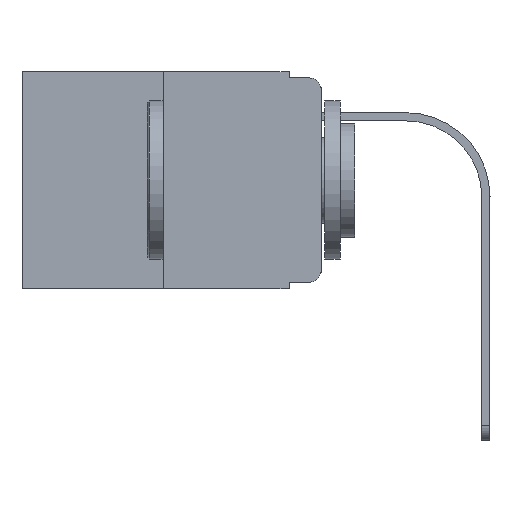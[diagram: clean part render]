
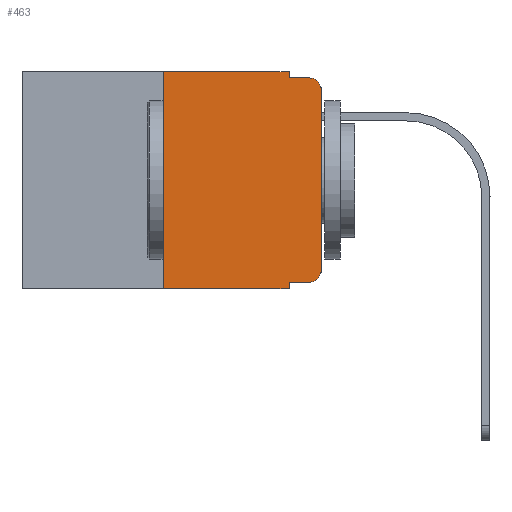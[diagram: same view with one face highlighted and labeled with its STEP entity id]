
A CAD part, left-side view. The second image highlights one B-rep face of the part: STEP entity #463.
In plain terms, the highlighted planar face has unit normal (-1, 0, 0).
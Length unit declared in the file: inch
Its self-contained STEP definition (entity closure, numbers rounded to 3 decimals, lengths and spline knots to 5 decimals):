
#173 = ORIENTED_EDGE ( 'NONE', *, *, #17405, .T. ) ;
#339 = DIRECTION ( 'NONE',  ( 0., 0., -1. ) ) ;
#370 = CARTESIAN_POINT ( 'NONE',  ( 0., 0.02, -0.333 ) ) ;
#463 = ADVANCED_FACE ( 'NONE', ( #6050 ), #9155, .F. ) ;
#794 = CARTESIAN_POINT ( 'NONE',  ( 0., 0.051, -0.343 ) ) ;
#1257 = VERTEX_POINT ( 'NONE', #794 ) ;
#1279 = DIRECTION ( 'NONE',  ( 0., 0., -1. ) ) ;
#1286 = VERTEX_POINT ( 'NONE', #20250 ) ;
#1422 = ORIENTED_EDGE ( 'NONE', *, *, #11324, .T. ) ;
#1457 = VERTEX_POINT ( 'NONE', #12810 ) ;
#1462 = AXIS2_PLACEMENT_3D ( 'NONE', #2928, #20805, #6211 ) ;
#1494 = VECTOR ( 'NONE', #10802, 39.37008 ) ;
#1573 = DIRECTION ( 'NONE',  ( 0., -1., 0. ) ) ;
#1656 = LINE ( 'NONE', #16146, #15437 ) ;
#2158 = ORIENTED_EDGE ( 'NONE', *, *, #18357, .F. ) ;
#2592 = VECTOR ( 'NONE', #14206, 39.37008 ) ;
#2595 = CARTESIAN_POINT ( 'NONE',  ( 0., 0.473, 0. ) ) ;
#2804 = VECTOR ( 'NONE', #20889, 39.37008 ) ;
#2928 = CARTESIAN_POINT ( 'NONE',  ( 0., 0.02, -0.313 ) ) ;
#2985 = AXIS2_PLACEMENT_3D ( 'NONE', #13853, #20326, #1279 ) ;
#3229 = ORIENTED_EDGE ( 'NONE', *, *, #9845, .F. ) ;
#3432 = LINE ( 'NONE', #14738, #16137 ) ;
#3999 = DIRECTION ( 'NONE',  ( 0., 0., -1. ) ) ;
#4090 = EDGE_LOOP ( 'NONE', ( #7844, #173, #4353, #8228, #8419, #2158, #6542, #3229, #13556, #1422 ) ) ;
#4353 = ORIENTED_EDGE ( 'NONE', *, *, #15361, .F. ) ;
#5995 = CARTESIAN_POINT ( 'NONE',  ( 0., 0.051, -0.333 ) ) ;
#6050 = FACE_OUTER_BOUND ( 'NONE', #4090, .T. ) ;
#6160 = VECTOR ( 'NONE', #3999, 39.37008 ) ;
#6211 = DIRECTION ( 'NONE',  ( 0., 0., -1. ) ) ;
#6542 = ORIENTED_EDGE ( 'NONE', *, *, #19393, .T. ) ;
#6975 = VECTOR ( 'NONE', #20547, 39.37008 ) ;
#7451 = CARTESIAN_POINT ( 'NONE',  ( 0., 0.051, 0. ) ) ;
#7591 = LINE ( 'NONE', #12385, #2592 ) ;
#7844 = ORIENTED_EDGE ( 'NONE', *, *, #13814, .T. ) ;
#8143 = DIRECTION ( 'NONE',  ( 0., 0., 1. ) ) ;
#8228 = ORIENTED_EDGE ( 'NONE', *, *, #18813, .F. ) ;
#8419 = ORIENTED_EDGE ( 'NONE', *, *, #12121, .F. ) ;
#8820 = VERTEX_POINT ( 'NONE', #16733 ) ;
#9155 = PLANE ( 'NONE',  #2985 ) ;
#9754 = VERTEX_POINT ( 'NONE', #5995 ) ;
#9845 = EDGE_CURVE ( 'NONE', #9754, #1257, #20593, .T. ) ;
#10029 = DIRECTION ( 'NONE',  ( -1., 0., 0. ) ) ;
#10431 = CIRCLE ( 'NONE', #11774, 0.02 ) ;
#10802 = DIRECTION ( 'NONE',  ( 0., -1., 0. ) ) ;
#10882 = CARTESIAN_POINT ( 'NONE',  ( 0., 0.25, 0. ) ) ;
#11324 = EDGE_CURVE ( 'NONE', #12050, #17138, #13033, .T. ) ;
#11774 = AXIS2_PLACEMENT_3D ( 'NONE', #18646, #10029, #339 ) ;
#12050 = VERTEX_POINT ( 'NONE', #370 ) ;
#12121 = EDGE_CURVE ( 'NONE', #14123, #12269, #13785, .T. ) ;
#12269 = VERTEX_POINT ( 'NONE', #18991 ) ;
#12385 = CARTESIAN_POINT ( 'NONE',  ( 0., 0.051, -0.333 ) ) ;
#12513 = CARTESIAN_POINT ( 'NONE',  ( 0., 0.051, 0. ) ) ;
#12573 = LINE ( 'NONE', #7451, #6975 ) ;
#12799 = VECTOR ( 'NONE', #1573, 39.37008 ) ;
#12810 = CARTESIAN_POINT ( 'NONE',  ( 0., 0.25, -0.343 ) ) ;
#13033 = CIRCLE ( 'NONE', #1462, 0.02 ) ;
#13131 = DIRECTION ( 'NONE',  ( 0., -1., 0. ) ) ;
#13556 = ORIENTED_EDGE ( 'NONE', *, *, #19650, .T. ) ;
#13785 = LINE ( 'NONE', #2595, #1494 ) ;
#13814 = EDGE_CURVE ( 'NONE', #17138, #8820, #1656, .T. ) ;
#13853 = CARTESIAN_POINT ( 'NONE',  ( 0., 0.473, 0. ) ) ;
#14123 = VERTEX_POINT ( 'NONE', #10882 ) ;
#14206 = DIRECTION ( 'NONE',  ( 0., -1., 0. ) ) ;
#14305 = CARTESIAN_POINT ( 'NONE',  ( 0., 0.25, 0. ) ) ;
#14494 = CARTESIAN_POINT ( 'NONE',  ( 0., 0.051, -0.01 ) ) ;
#14738 = CARTESIAN_POINT ( 'NONE',  ( 0., 0.051, -0.01 ) ) ;
#15361 = EDGE_CURVE ( 'NONE', #18995, #1286, #3432, .T. ) ;
#15437 = VECTOR ( 'NONE', #8143, 39.37008 ) ;
#16137 = VECTOR ( 'NONE', #13131, 39.37008 ) ;
#16146 = CARTESIAN_POINT ( 'NONE',  ( 0., 0., 0. ) ) ;
#16220 = CARTESIAN_POINT ( 'NONE',  ( 0., 0., -0.313 ) ) ;
#16733 = CARTESIAN_POINT ( 'NONE',  ( 0., 0., -0.03 ) ) ;
#17138 = VERTEX_POINT ( 'NONE', #16220 ) ;
#17405 = EDGE_CURVE ( 'NONE', #8820, #1286, #10431, .T. ) ;
#17656 = LINE ( 'NONE', #17857, #12799 ) ;
#17857 = CARTESIAN_POINT ( 'NONE',  ( 0., 0.473, -0.343 ) ) ;
#18357 = EDGE_CURVE ( 'NONE', #1457, #14123, #19199, .T. ) ;
#18646 = CARTESIAN_POINT ( 'NONE',  ( 0., 0.02, -0.03 ) ) ;
#18813 = EDGE_CURVE ( 'NONE', #12269, #18995, #12573, .T. ) ;
#18991 = CARTESIAN_POINT ( 'NONE',  ( 0., 0.051, 0. ) ) ;
#18995 = VERTEX_POINT ( 'NONE', #14494 ) ;
#19199 = LINE ( 'NONE', #14305, #2804 ) ;
#19393 = EDGE_CURVE ( 'NONE', #1457, #1257, #17656, .T. ) ;
#19650 = EDGE_CURVE ( 'NONE', #9754, #12050, #7591, .T. ) ;
#20250 = CARTESIAN_POINT ( 'NONE',  ( 0., 0.02, -0.01 ) ) ;
#20326 = DIRECTION ( 'NONE',  ( 1., 0., 0. ) ) ;
#20547 = DIRECTION ( 'NONE',  ( 0., 0., -1. ) ) ;
#20593 = LINE ( 'NONE', #12513, #6160 ) ;
#20805 = DIRECTION ( 'NONE',  ( -1., 0., 0. ) ) ;
#20889 = DIRECTION ( 'NONE',  ( 0., 0., 1. ) ) ;
